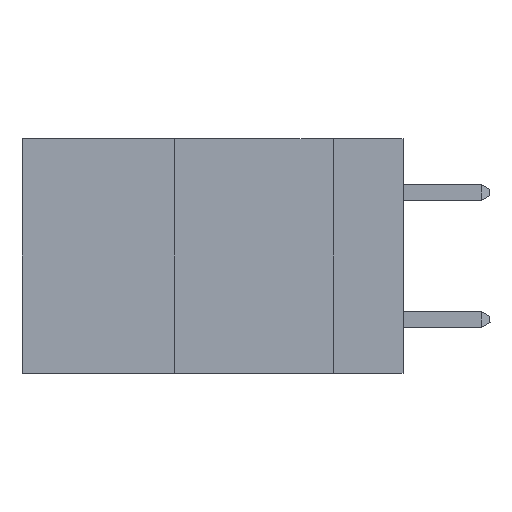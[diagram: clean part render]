
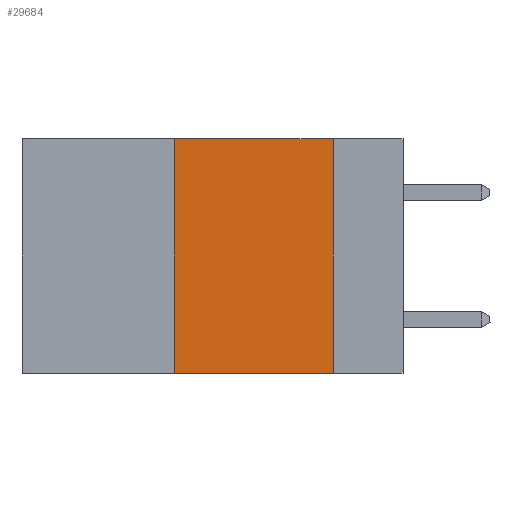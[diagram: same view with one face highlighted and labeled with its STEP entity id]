
A CAD part, left-side view. The second image highlights one B-rep face of the part: STEP entity #29684.
In plain terms, the highlighted planar face has unit normal (-1, 0, 0).
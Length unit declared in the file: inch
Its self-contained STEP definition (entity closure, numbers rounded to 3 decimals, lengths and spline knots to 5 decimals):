
#2020 = LINE ( 'NONE', #18885, #2950 ) ;
#2950 = VECTOR ( 'NONE', #21900, 39.37008 ) ;
#3224 = ORIENTED_EDGE ( 'NONE', *, *, #26983, .F. ) ;
#3228 = DIRECTION ( 'NONE',  ( 0., 0., 1. ) ) ;
#3767 = VERTEX_POINT ( 'NONE', #11493 ) ;
#6524 = CARTESIAN_POINT ( 'NONE',  ( 0., 0.6, 0. ) ) ;
#7051 = PLANE ( 'NONE',  #28381 ) ;
#7134 = ORIENTED_EDGE ( 'NONE', *, *, #28246, .F. ) ;
#7153 = VECTOR ( 'NONE', #3228, 39.37008 ) ;
#8947 = EDGE_CURVE ( 'NONE', #3767, #22240, #10963, .T. ) ;
#10650 = LINE ( 'NONE', #22830, #38035 ) ;
#10963 = LINE ( 'NONE', #21584, #7153 ) ;
#11493 = CARTESIAN_POINT ( 'NONE',  ( 0., 0.36, -0.37 ) ) ;
#12532 = VECTOR ( 'NONE', #12555, 39.37008 ) ;
#12555 = DIRECTION ( 'NONE',  ( 0., 0., -1. ) ) ;
#15759 = CARTESIAN_POINT ( 'NONE',  ( 0., 0.11, 0. ) ) ;
#18630 = CARTESIAN_POINT ( 'NONE',  ( 0., 0.36, 0. ) ) ;
#18885 = CARTESIAN_POINT ( 'NONE',  ( 0., 0.6, 0. ) ) ;
#20557 = ORIENTED_EDGE ( 'NONE', *, *, #8947, .F. ) ;
#20850 = EDGE_LOOP ( 'NONE', ( #3224, #7134, #20557, #39033 ) ) ;
#21584 = CARTESIAN_POINT ( 'NONE',  ( 0., 0.36, 0. ) ) ;
#21900 = DIRECTION ( 'NONE',  ( 0., -1., 0. ) ) ;
#22240 = VERTEX_POINT ( 'NONE', #18630 ) ;
#22830 = CARTESIAN_POINT ( 'NONE',  ( 0., 0.6, -0.37 ) ) ;
#24343 = VERTEX_POINT ( 'NONE', #24684 ) ;
#24684 = CARTESIAN_POINT ( 'NONE',  ( 0., 0.11, -0.37 ) ) ;
#25597 = LINE ( 'NONE', #15759, #12532 ) ;
#26832 = FACE_OUTER_BOUND ( 'NONE', #20850, .T. ) ;
#26983 = EDGE_CURVE ( 'NONE', #32122, #24343, #25597, .T. ) ;
#27723 = CARTESIAN_POINT ( 'NONE',  ( 0., 0.11, 0. ) ) ;
#27979 = DIRECTION ( 'NONE',  ( 1., 0., 0. ) ) ;
#28246 = EDGE_CURVE ( 'NONE', #22240, #32122, #2020, .T. ) ;
#28381 = AXIS2_PLACEMENT_3D ( 'NONE', #6524, #27979, #37492 ) ;
#29135 = DIRECTION ( 'NONE',  ( 0., -1., 0. ) ) ;
#29684 = ADVANCED_FACE ( 'NONE', ( #26832 ), #7051, .F. ) ;
#32122 = VERTEX_POINT ( 'NONE', #27723 ) ;
#36525 = EDGE_CURVE ( 'NONE', #3767, #24343, #10650, .T. ) ;
#37492 = DIRECTION ( 'NONE',  ( 0., 0., -1. ) ) ;
#38035 = VECTOR ( 'NONE', #29135, 39.37008 ) ;
#39033 = ORIENTED_EDGE ( 'NONE', *, *, #36525, .T. ) ;
